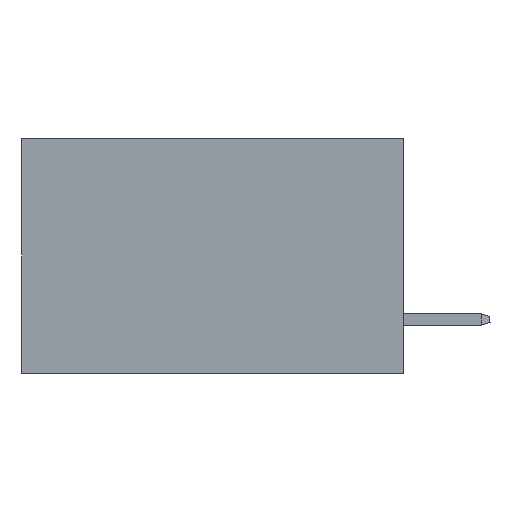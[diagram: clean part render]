
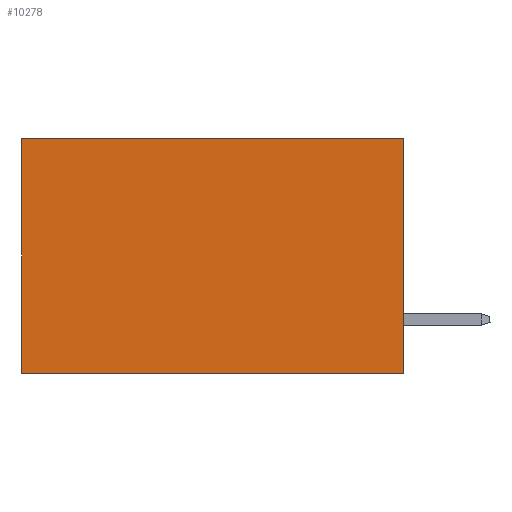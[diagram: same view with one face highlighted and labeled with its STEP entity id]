
A CAD part, left-side view. The second image highlights one B-rep face of the part: STEP entity #10278.
In plain terms, the highlighted planar face has unit normal (-1, 0, 0).
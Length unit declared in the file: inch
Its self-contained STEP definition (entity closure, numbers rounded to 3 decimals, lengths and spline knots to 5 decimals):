
#1280 = VECTOR ( 'NONE', #2401, 39.37008 ) ;
#1571 = FACE_OUTER_BOUND ( 'NONE', #24702, .T. ) ;
#2401 = DIRECTION ( 'NONE',  ( 0., 0., -1. ) ) ;
#3318 = EDGE_CURVE ( 'NONE', #25922, #6741, #22498, .T. ) ;
#4603 = CARTESIAN_POINT ( 'NONE',  ( 0.2875, 0., 0. ) ) ;
#4657 = VECTOR ( 'NONE', #12600, 39.37008 ) ;
#5171 = LINE ( 'NONE', #27710, #18490 ) ;
#6260 = CARTESIAN_POINT ( 'NONE',  ( 0.2875, 0., 0. ) ) ;
#6741 = VERTEX_POINT ( 'NONE', #15559 ) ;
#7015 = ORIENTED_EDGE ( 'NONE', *, *, #3318, .F. ) ;
#7293 = EDGE_CURVE ( 'NONE', #6741, #14269, #10382, .T. ) ;
#8849 = CARTESIAN_POINT ( 'NONE',  ( 0.2875, 0.6, 0. ) ) ;
#10278 = ADVANCED_FACE ( 'NONE', ( #1571 ), #28642, .F. ) ;
#10382 = LINE ( 'NONE', #28083, #4657 ) ;
#10655 = DIRECTION ( 'NONE',  ( 1., 0., 0. ) ) ;
#12600 = DIRECTION ( 'NONE',  ( 0., 1., 0. ) ) ;
#12625 = CARTESIAN_POINT ( 'NONE',  ( 0.2875, 0., 0. ) ) ;
#14201 = VECTOR ( 'NONE', #24689, 39.37008 ) ;
#14269 = VERTEX_POINT ( 'NONE', #20169 ) ;
#15487 = DIRECTION ( 'NONE',  ( 0., 0., -1. ) ) ;
#15492 = VERTEX_POINT ( 'NONE', #8849 ) ;
#15559 = CARTESIAN_POINT ( 'NONE',  ( 0.2875, 0., -0.37 ) ) ;
#16076 = ORIENTED_EDGE ( 'NONE', *, *, #7293, .F. ) ;
#18490 = VECTOR ( 'NONE', #25225, 39.37008 ) ;
#20106 = ORIENTED_EDGE ( 'NONE', *, *, #20621, .T. ) ;
#20169 = CARTESIAN_POINT ( 'NONE',  ( 0.2875, 0.6, -0.37 ) ) ;
#20621 = EDGE_CURVE ( 'NONE', #25922, #15492, #27420, .T. ) ;
#22498 = LINE ( 'NONE', #4603, #1280 ) ;
#22691 = ORIENTED_EDGE ( 'NONE', *, *, #26698, .T. ) ;
#24689 = DIRECTION ( 'NONE',  ( 0., 1., 0. ) ) ;
#24702 = EDGE_LOOP ( 'NONE', ( #22691, #16076, #7015, #20106 ) ) ;
#25225 = DIRECTION ( 'NONE',  ( 0., 0., -1. ) ) ;
#25383 = CARTESIAN_POINT ( 'NONE',  ( 0.2875, 0., 0. ) ) ;
#25922 = VERTEX_POINT ( 'NONE', #12625 ) ;
#26698 = EDGE_CURVE ( 'NONE', #15492, #14269, #5171, .T. ) ;
#27420 = LINE ( 'NONE', #25383, #14201 ) ;
#27710 = CARTESIAN_POINT ( 'NONE',  ( 0.2875, 0.6, 0. ) ) ;
#28083 = CARTESIAN_POINT ( 'NONE',  ( 0.2875, 0., -0.37 ) ) ;
#28298 = AXIS2_PLACEMENT_3D ( 'NONE', #6260, #10655, #15487 ) ;
#28642 = PLANE ( 'NONE',  #28298 ) ;
